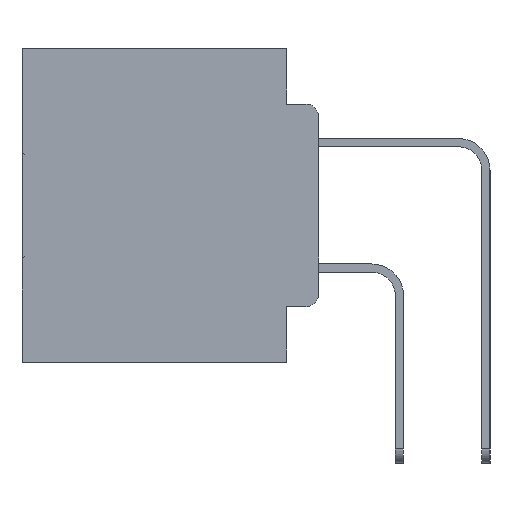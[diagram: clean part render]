
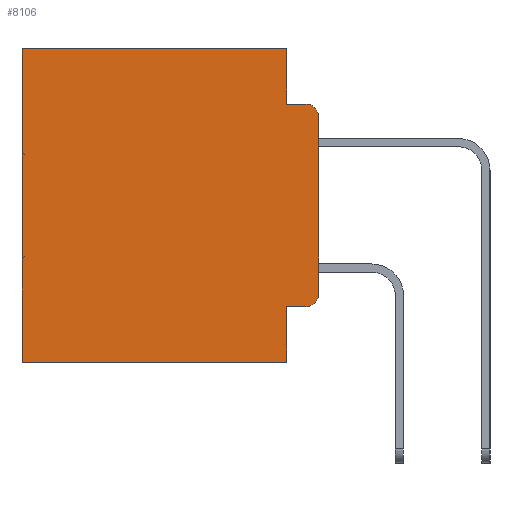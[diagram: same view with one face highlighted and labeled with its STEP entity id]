
A CAD part, left-side view. The second image highlights one B-rep face of the part: STEP entity #8106.
In plain terms, the highlighted planar face has unit normal (-1, 0, 0).
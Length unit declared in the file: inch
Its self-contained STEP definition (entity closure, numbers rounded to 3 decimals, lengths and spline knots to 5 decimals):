
#261 = CIRCLE ( 'NONE', #26006, 0.02 ) ;
#347 = EDGE_CURVE ( 'NONE', #15738, #20896, #18889, .T. ) ;
#550 = EDGE_LOOP ( 'NONE', ( #28844, #32460, #33256, #9431, #13066, #19373, #4364, #17781, #9217, #17355 ) ) ;
#1093 = EDGE_CURVE ( 'NONE', #11607, #23611, #23635, .T. ) ;
#1176 = VECTOR ( 'NONE', #22992, 39.37008 ) ;
#1348 = DIRECTION ( 'NONE',  ( 0., 0., -1. ) ) ;
#1612 = VERTEX_POINT ( 'NONE', #31662 ) ;
#1954 = CARTESIAN_POINT ( 'NONE',  ( 0.298, 0.051, -0.4115 ) ) ;
#2317 = PLANE ( 'NONE',  #13167 ) ;
#4038 = CARTESIAN_POINT ( 'NONE',  ( 0.298, 0., -0.5 ) ) ;
#4272 = VECTOR ( 'NONE', #15257, 39.37008 ) ;
#4364 = ORIENTED_EDGE ( 'NONE', *, *, #7881, .F. ) ;
#4417 = EDGE_CURVE ( 'NONE', #11607, #7697, #15013, .T. ) ;
#4545 = CARTESIAN_POINT ( 'NONE',  ( 0.298, 0.473, 0. ) ) ;
#4690 = VECTOR ( 'NONE', #12669, 39.37008 ) ;
#4764 = VERTEX_POINT ( 'NONE', #30529 ) ;
#6867 = DIRECTION ( 'NONE',  ( -1., 0., 0. ) ) ;
#7697 = VERTEX_POINT ( 'NONE', #26348 ) ;
#7881 = EDGE_CURVE ( 'NONE', #7697, #1612, #26551, .T. ) ;
#8106 = ADVANCED_FACE ( 'NONE', ( #26936 ), #2317, .F. ) ;
#8656 = CARTESIAN_POINT ( 'NONE',  ( 0.298, 0.051, 0. ) ) ;
#9124 = CARTESIAN_POINT ( 'NONE',  ( 0.298, 0.473, 0. ) ) ;
#9217 = ORIENTED_EDGE ( 'NONE', *, *, #1093, .T. ) ;
#9431 = ORIENTED_EDGE ( 'NONE', *, *, #347, .F. ) ;
#9957 = CARTESIAN_POINT ( 'NONE',  ( 0.298, 0.051, -0.0885 ) ) ;
#10002 = VERTEX_POINT ( 'NONE', #14874 ) ;
#11416 = CARTESIAN_POINT ( 'NONE',  ( 0.298, 0., 0. ) ) ;
#11605 = LINE ( 'NONE', #28113, #4690 ) ;
#11607 = VERTEX_POINT ( 'NONE', #23876 ) ;
#11883 = DIRECTION ( 'NONE',  ( 0., 1., 0. ) ) ;
#12669 = DIRECTION ( 'NONE',  ( 0., -1., 0. ) ) ;
#13066 = ORIENTED_EDGE ( 'NONE', *, *, #21245, .T. ) ;
#13167 = AXIS2_PLACEMENT_3D ( 'NONE', #33290, #33403, #18014 ) ;
#14011 = DIRECTION ( 'NONE',  ( 0., 1., 0. ) ) ;
#14233 = DIRECTION ( 'NONE',  ( 0., 0., -1. ) ) ;
#14874 = CARTESIAN_POINT ( 'NONE',  ( 0.298, 0., -0.1085 ) ) ;
#15013 = LINE ( 'NONE', #8656, #29515 ) ;
#15257 = DIRECTION ( 'NONE',  ( 0., 0., -1. ) ) ;
#15738 = VERTEX_POINT ( 'NONE', #23480 ) ;
#16009 = EDGE_CURVE ( 'NONE', #18222, #1612, #24802, .T. ) ;
#16374 = VECTOR ( 'NONE', #14233, 39.37008 ) ;
#16487 = CARTESIAN_POINT ( 'NONE',  ( 0.298, 0.051, 0. ) ) ;
#16934 = DIRECTION ( 'NONE',  ( -1., 0., 0. ) ) ;
#17136 = DIRECTION ( 'NONE',  ( 0., -1., 0. ) ) ;
#17355 = ORIENTED_EDGE ( 'NONE', *, *, #25468, .T. ) ;
#17781 = ORIENTED_EDGE ( 'NONE', *, *, #4417, .F. ) ;
#18014 = DIRECTION ( 'NONE',  ( 0., 0., -1. ) ) ;
#18222 = VERTEX_POINT ( 'NONE', #4545 ) ;
#18889 = LINE ( 'NONE', #16487, #4272 ) ;
#19373 = ORIENTED_EDGE ( 'NONE', *, *, #16009, .T. ) ;
#20407 = CIRCLE ( 'NONE', #30765, 0.02 ) ;
#20415 = CARTESIAN_POINT ( 'NONE',  ( 0.298, 0., 0. ) ) ;
#20896 = VERTEX_POINT ( 'NONE', #9957 ) ;
#21245 = EDGE_CURVE ( 'NONE', #15738, #18222, #21583, .T. ) ;
#21583 = LINE ( 'NONE', #11416, #27647 ) ;
#22328 = CARTESIAN_POINT ( 'NONE',  ( 0.298, 0.02, -0.1085 ) ) ;
#22992 = DIRECTION ( 'NONE',  ( 0., 0., -1. ) ) ;
#23356 = EDGE_CURVE ( 'NONE', #10002, #4764, #28708, .T. ) ;
#23480 = CARTESIAN_POINT ( 'NONE',  ( 0.298, 0.051, 0. ) ) ;
#23611 = VERTEX_POINT ( 'NONE', #29616 ) ;
#23635 = LINE ( 'NONE', #1954, #29698 ) ;
#23876 = CARTESIAN_POINT ( 'NONE',  ( 0.298, 0.051, -0.4115 ) ) ;
#24802 = LINE ( 'NONE', #9124, #16374 ) ;
#24928 = DIRECTION ( 'NONE',  ( 0., 0., -1. ) ) ;
#25468 = EDGE_CURVE ( 'NONE', #23611, #4764, #261, .T. ) ;
#25968 = CARTESIAN_POINT ( 'NONE',  ( 0.298, 0.02, -0.0885 ) ) ;
#26006 = AXIS2_PLACEMENT_3D ( 'NONE', #32323, #16934, #1348 ) ;
#26348 = CARTESIAN_POINT ( 'NONE',  ( 0.298, 0.051, -0.5 ) ) ;
#26404 = EDGE_CURVE ( 'NONE', #20896, #27612, #11605, .T. ) ;
#26551 = LINE ( 'NONE', #4038, #31776 ) ;
#26740 = DIRECTION ( 'NONE',  ( 0., 0., -1. ) ) ;
#26936 = FACE_OUTER_BOUND ( 'NONE', #550, .T. ) ;
#27473 = EDGE_CURVE ( 'NONE', #10002, #27612, #20407, .T. ) ;
#27612 = VERTEX_POINT ( 'NONE', #25968 ) ;
#27647 = VECTOR ( 'NONE', #14011, 39.37008 ) ;
#28113 = CARTESIAN_POINT ( 'NONE',  ( 0.298, 0.051, -0.0885 ) ) ;
#28708 = LINE ( 'NONE', #20415, #1176 ) ;
#28844 = ORIENTED_EDGE ( 'NONE', *, *, #23356, .F. ) ;
#29515 = VECTOR ( 'NONE', #26740, 39.37008 ) ;
#29616 = CARTESIAN_POINT ( 'NONE',  ( 0.298, 0.02, -0.4115 ) ) ;
#29698 = VECTOR ( 'NONE', #17136, 39.37008 ) ;
#30529 = CARTESIAN_POINT ( 'NONE',  ( 0.298, 0., -0.3915 ) ) ;
#30765 = AXIS2_PLACEMENT_3D ( 'NONE', #22328, #6867, #24928 ) ;
#31662 = CARTESIAN_POINT ( 'NONE',  ( 0.298, 0.473, -0.5 ) ) ;
#31776 = VECTOR ( 'NONE', #11883, 39.37008 ) ;
#32323 = CARTESIAN_POINT ( 'NONE',  ( 0.298, 0.02, -0.3915 ) ) ;
#32460 = ORIENTED_EDGE ( 'NONE', *, *, #27473, .T. ) ;
#33256 = ORIENTED_EDGE ( 'NONE', *, *, #26404, .F. ) ;
#33290 = CARTESIAN_POINT ( 'NONE',  ( 0.298, 0., 0. ) ) ;
#33403 = DIRECTION ( 'NONE',  ( 1., 0., 0. ) ) ;
